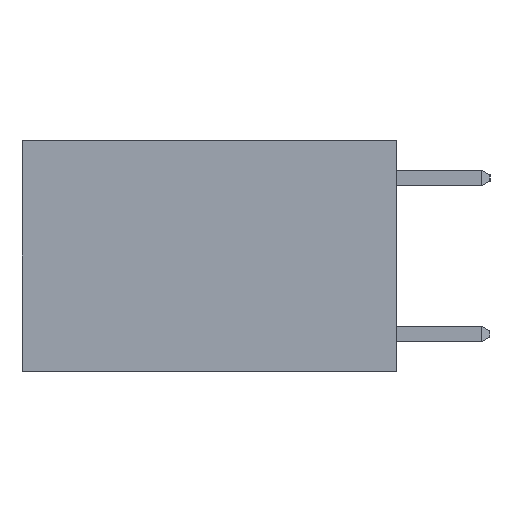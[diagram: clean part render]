
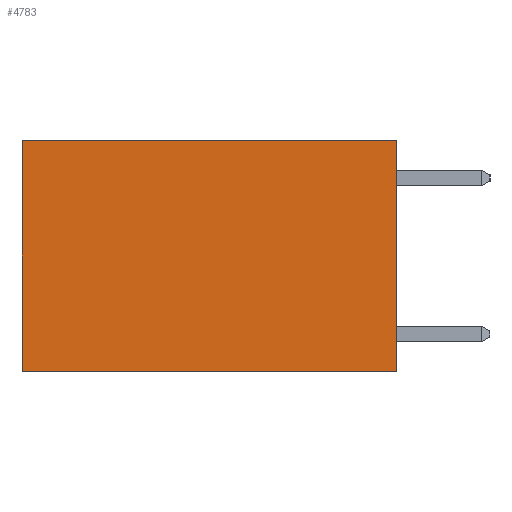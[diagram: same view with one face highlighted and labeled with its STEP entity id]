
A CAD part, left-side view. The second image highlights one B-rep face of the part: STEP entity #4783.
In plain terms, the highlighted planar face has unit normal (-1, 0, 0).
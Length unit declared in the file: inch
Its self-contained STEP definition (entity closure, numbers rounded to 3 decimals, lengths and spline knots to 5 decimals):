
#159 = LINE ( 'NONE', #9317, #6799 ) ;
#504 = VERTEX_POINT ( 'NONE', #8152 ) ;
#560 = EDGE_CURVE ( 'NONE', #6023, #8475, #3775, .T. ) ;
#671 = VECTOR ( 'NONE', #1746, 39.37008 ) ;
#1554 = AXIS2_PLACEMENT_3D ( 'NONE', #8447, #9263, #4201 ) ;
#1746 = DIRECTION ( 'NONE',  ( 0., 1., 0. ) ) ;
#2345 = FACE_OUTER_BOUND ( 'NONE', #2360, .T. ) ;
#2360 = EDGE_LOOP ( 'NONE', ( #8588, #4322, #6711, #8844 ) ) ;
#2499 = CARTESIAN_POINT ( 'NONE',  ( 0.2625, 0., -0.37 ) ) ;
#3775 = LINE ( 'NONE', #8054, #10250 ) ;
#4201 = DIRECTION ( 'NONE',  ( 0., 0., -1. ) ) ;
#4322 = ORIENTED_EDGE ( 'NONE', *, *, #560, .F. ) ;
#4430 = VERTEX_POINT ( 'NONE', #9768 ) ;
#4783 = ADVANCED_FACE ( 'NONE', ( #2345 ), #7658, .F. ) ;
#4856 = DIRECTION ( 'NONE',  ( 0., 1., 0. ) ) ;
#5375 = EDGE_CURVE ( 'NONE', #4430, #8475, #159, .T. ) ;
#5611 = LINE ( 'NONE', #10193, #671 ) ;
#6023 = VERTEX_POINT ( 'NONE', #2499 ) ;
#6073 = EDGE_CURVE ( 'NONE', #504, #4430, #5611, .T. ) ;
#6711 = ORIENTED_EDGE ( 'NONE', *, *, #8456, .F. ) ;
#6799 = VECTOR ( 'NONE', #7746, 39.37008 ) ;
#7539 = VECTOR ( 'NONE', #10157, 39.37008 ) ;
#7658 = PLANE ( 'NONE',  #1554 ) ;
#7746 = DIRECTION ( 'NONE',  ( 0., 0., -1. ) ) ;
#7813 = CARTESIAN_POINT ( 'NONE',  ( 0.2625, 0.6, -0.37 ) ) ;
#8054 = CARTESIAN_POINT ( 'NONE',  ( 0.2625, 0., -0.37 ) ) ;
#8152 = CARTESIAN_POINT ( 'NONE',  ( 0.2625, 0., 0. ) ) ;
#8447 = CARTESIAN_POINT ( 'NONE',  ( 0.2625, 0., 0. ) ) ;
#8456 = EDGE_CURVE ( 'NONE', #504, #6023, #9674, .T. ) ;
#8475 = VERTEX_POINT ( 'NONE', #7813 ) ;
#8588 = ORIENTED_EDGE ( 'NONE', *, *, #5375, .T. ) ;
#8592 = CARTESIAN_POINT ( 'NONE',  ( 0.2625, 0., 0. ) ) ;
#8844 = ORIENTED_EDGE ( 'NONE', *, *, #6073, .T. ) ;
#9263 = DIRECTION ( 'NONE',  ( 1., 0., 0. ) ) ;
#9317 = CARTESIAN_POINT ( 'NONE',  ( 0.2625, 0.6, 0. ) ) ;
#9674 = LINE ( 'NONE', #8592, #7539 ) ;
#9768 = CARTESIAN_POINT ( 'NONE',  ( 0.2625, 0.6, 0. ) ) ;
#10157 = DIRECTION ( 'NONE',  ( 0., 0., -1. ) ) ;
#10193 = CARTESIAN_POINT ( 'NONE',  ( 0.2625, 0., 0. ) ) ;
#10250 = VECTOR ( 'NONE', #4856, 39.37008 ) ;
